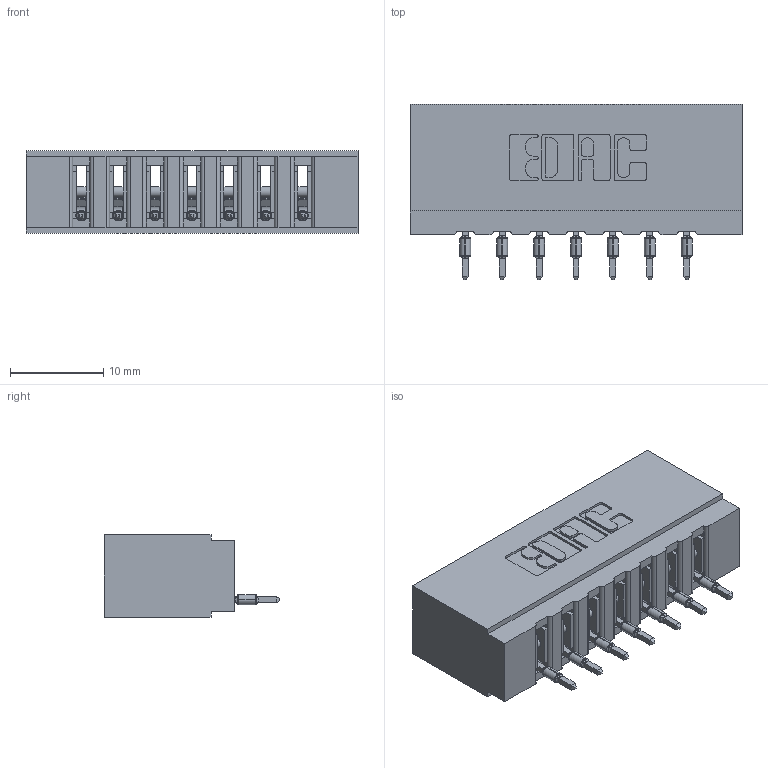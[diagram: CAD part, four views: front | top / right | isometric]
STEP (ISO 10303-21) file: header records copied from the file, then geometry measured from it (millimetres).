
FILE_DESCRIPTION (( 'STEP AP203' ), '1' );
FILE_NAME ('717-007-560-106.STEP', '2020-03-13T17:44:22', ( '' ), ( '' ), 'SwSTEP 2.0', 'SolidWorks 2016', '' );
FILE_SCHEMA (( 'CONFIG_CONTROL_DESIGN' ));
Length unit declared in the file: inch
Products named in the file (3): 717-007-560-106; 745-292-001_560; 717 Part_Insulator Option - 06
Assembly tree (8 placements, depth 2):
  717-007-560-106
    717 Part_Insulator Option - 06
    745-292-001_560  x7
Bounding box: 35.61 x 18.78 x 8.89 mm (x, y, z)
Volume: 3187.7 mm3; surface area: 4210.4 mm2
Topology: 8 solids, 8 shells, 948 faces, 2631 edges, 1678 vertices
Faces by surface type: plane 565, cylinder 201, bspline 140, torus 42
Entity records: 16830 total; most frequent: CARTESIAN_POINT 3466, ORIENTED_EDGE 2838, DIRECTION 2501, EDGE_CURVE 1419, LINE 1187, VECTOR 1187, VERTEX_POINT 910, AXIS2_PLACEMENT_3D 657
